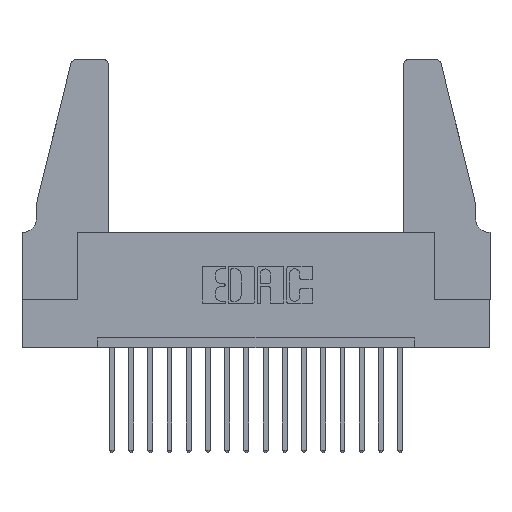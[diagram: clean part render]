
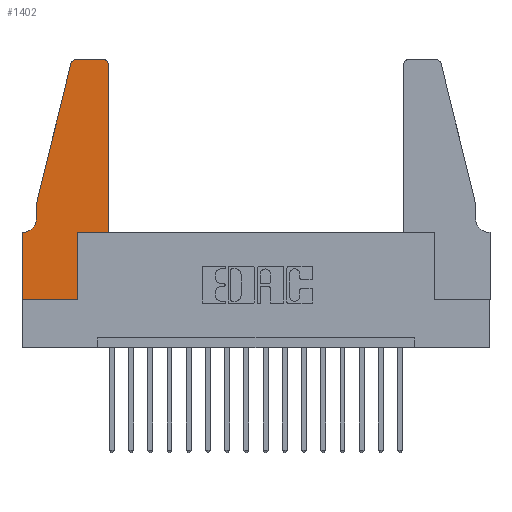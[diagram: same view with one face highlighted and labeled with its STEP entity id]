
A CAD part, top view. The second image highlights one B-rep face of the part: STEP entity #1402.
In plain terms, the highlighted planar face has unit normal (0, 0, 1).
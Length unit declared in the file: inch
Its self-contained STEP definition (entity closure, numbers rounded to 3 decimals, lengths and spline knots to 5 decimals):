
#218 = CARTESIAN_POINT ( 'NONE',  ( 0.25487, 1.22718, 0.37 ) ) ;
#246 = CIRCLE ( 'NONE', #5915, 0.03 ) ;
#632 = CARTESIAN_POINT ( 'NONE',  ( 0.4505, 0.35, 0.37 ) ) ;
#661 = LINE ( 'NONE', #895, #12252 ) ;
#686 = DIRECTION ( 'NONE',  ( -1., 0., 0. ) ) ;
#746 = DIRECTION ( 'NONE',  ( 1., 0., 0. ) ) ;
#895 = CARTESIAN_POINT ( 'NONE',  ( 0.0755, 0.35, 0.37 ) ) ;
#911 = VERTEX_POINT ( 'NONE', #13618 ) ;
#955 = CARTESIAN_POINT ( 'NONE',  ( 0.4205, 1.25, 0.37 ) ) ;
#1237 = CARTESIAN_POINT ( 'NONE',  ( 0.2865, 0.35, 0.37 ) ) ;
#1300 = DIRECTION ( 'NONE',  ( 0., 1., 0. ) ) ;
#1331 = EDGE_CURVE ( 'NONE', #10285, #3420, #5585, .T. ) ;
#1402 = ADVANCED_FACE ( 'NONE', ( #6008 ), #6118, .T. ) ;
#1501 = AXIS2_PLACEMENT_3D ( 'NONE', #3945, #5365, #5614 ) ;
#1996 = CARTESIAN_POINT ( 'NONE',  ( 0.0055, 0.42, 0.37 ) ) ;
#2020 = LINE ( 'NONE', #7307, #12555 ) ;
#3420 = VERTEX_POINT ( 'NONE', #8411 ) ;
#3944 = EDGE_CURVE ( 'NONE', #3420, #10377, #2020, .T. ) ;
#3945 = CARTESIAN_POINT ( 'NONE',  ( 0.284, 1.22, 0.37 ) ) ;
#4364 = DIRECTION ( 'NONE',  ( 0., -1., 0. ) ) ;
#4513 = VERTEX_POINT ( 'NONE', #7907 ) ;
#4606 = DIRECTION ( 'NONE',  ( 1., 0., 0. ) ) ;
#4682 = VERTEX_POINT ( 'NONE', #5174 ) ;
#4946 = EDGE_CURVE ( 'NONE', #10165, #10457, #15921, .T. ) ;
#5174 = CARTESIAN_POINT ( 'NONE',  ( 0.4505, 1.22, 0.37 ) ) ;
#5352 = VERTEX_POINT ( 'NONE', #11064 ) ;
#5365 = DIRECTION ( 'NONE',  ( 0., 0., 1. ) ) ;
#5369 = LINE ( 'NONE', #7234, #12212 ) ;
#5465 = ORIENTED_EDGE ( 'NONE', *, *, #4946, .T. ) ;
#5471 = VERTEX_POINT ( 'NONE', #955 ) ;
#5585 = LINE ( 'NONE', #10132, #12208 ) ;
#5614 = DIRECTION ( 'NONE',  ( 1., 0., 0. ) ) ;
#5915 = AXIS2_PLACEMENT_3D ( 'NONE', #13156, #6268, #15820 ) ;
#5952 = DIRECTION ( 'NONE',  ( -1., 0., 0. ) ) ;
#5994 = VERTEX_POINT ( 'NONE', #632 ) ;
#6008 = FACE_OUTER_BOUND ( 'NONE', #15232, .T. ) ;
#6050 = DIRECTION ( 'NONE',  ( 0., -1., 0. ) ) ;
#6091 = EDGE_CURVE ( 'NONE', #4513, #5352, #15668, .T. ) ;
#6118 = PLANE ( 'NONE',  #15606 ) ;
#6236 = DIRECTION ( 'NONE',  ( 0., 0., -1. ) ) ;
#6268 = DIRECTION ( 'NONE',  ( 0., 0., 1. ) ) ;
#6498 = LINE ( 'NONE', #13769, #12497 ) ;
#7151 = CARTESIAN_POINT ( 'NONE',  ( 0.0755, 0.5, 0.37 ) ) ;
#7234 = CARTESIAN_POINT ( 'NONE',  ( 0.2605, 1.25, 0.37 ) ) ;
#7270 = EDGE_CURVE ( 'NONE', #4682, #5471, #246, .T. ) ;
#7307 = CARTESIAN_POINT ( 'NONE',  ( 0., 0., 0.37 ) ) ;
#7512 = ORIENTED_EDGE ( 'NONE', *, *, #15019, .T. ) ;
#7577 = CARTESIAN_POINT ( 'NONE',  ( 0., 0.35, 0.37 ) ) ;
#7890 = ORIENTED_EDGE ( 'NONE', *, *, #8281, .T. ) ;
#7907 = CARTESIAN_POINT ( 'NONE',  ( 0.0755, 0.5, 0.37 ) ) ;
#8196 = ORIENTED_EDGE ( 'NONE', *, *, #8387, .T. ) ;
#8281 = EDGE_CURVE ( 'NONE', #5471, #10165, #5369, .T. ) ;
#8378 = VECTOR ( 'NONE', #6050, 39.37008 ) ;
#8387 = EDGE_CURVE ( 'NONE', #9005, #5994, #14546, .T. ) ;
#8411 = CARTESIAN_POINT ( 'NONE',  ( 0., 0., 0.37 ) ) ;
#8849 = CARTESIAN_POINT ( 'NONE',  ( 0.4505, 0.35, 0.37 ) ) ;
#8960 = DIRECTION ( 'NONE',  ( 0., 0., 1. ) ) ;
#9005 = VERTEX_POINT ( 'NONE', #15796 ) ;
#9134 = CARTESIAN_POINT ( 'NONE',  ( 0.284, 1.25, 0.37 ) ) ;
#9486 = CARTESIAN_POINT ( 'NONE',  ( 0.2865, 0., 0.37 ) ) ;
#9687 = DIRECTION ( 'NONE',  ( 0., 1., 0. ) ) ;
#10042 = ORIENTED_EDGE ( 'NONE', *, *, #16194, .T. ) ;
#10132 = CARTESIAN_POINT ( 'NONE',  ( 0., 0., 0.37 ) ) ;
#10165 = VERTEX_POINT ( 'NONE', #9134 ) ;
#10285 = VERTEX_POINT ( 'NONE', #12871 ) ;
#10377 = VERTEX_POINT ( 'NONE', #9486 ) ;
#10457 = VERTEX_POINT ( 'NONE', #218 ) ;
#10514 = LINE ( 'NONE', #17068, #16288 ) ;
#10724 = ORIENTED_EDGE ( 'NONE', *, *, #15598, .T. ) ;
#10928 = VECTOR ( 'NONE', #4606, 39.37008 ) ;
#11064 = CARTESIAN_POINT ( 'NONE',  ( 0.0755, 0.42, 0.37 ) ) ;
#11336 = VECTOR ( 'NONE', #1300, 39.37008 ) ;
#11367 = ORIENTED_EDGE ( 'NONE', *, *, #7270, .T. ) ;
#11774 = LINE ( 'NONE', #1237, #11336 ) ;
#12208 = VECTOR ( 'NONE', #4364, 39.37008 ) ;
#12212 = VECTOR ( 'NONE', #5952, 39.37008 ) ;
#12252 = VECTOR ( 'NONE', #13246, 39.37008 ) ;
#12497 = VECTOR ( 'NONE', #9687, 39.37008 ) ;
#12555 = VECTOR ( 'NONE', #14224, 39.37008 ) ;
#12871 = CARTESIAN_POINT ( 'NONE',  ( 0., 0.35, 0.37 ) ) ;
#13049 = ORIENTED_EDGE ( 'NONE', *, *, #6091, .T. ) ;
#13156 = CARTESIAN_POINT ( 'NONE',  ( 0.4205, 1.22, 0.37 ) ) ;
#13246 = DIRECTION ( 'NONE',  ( -1., 0., 0. ) ) ;
#13420 = AXIS2_PLACEMENT_3D ( 'NONE', #1996, #6236, #686 ) ;
#13618 = CARTESIAN_POINT ( 'NONE',  ( 0.0055, 0.35, 0.37 ) ) ;
#13760 = CIRCLE ( 'NONE', #13420, 0.07 ) ;
#13769 = CARTESIAN_POINT ( 'NONE',  ( 0.4505, 0.35, 0.37 ) ) ;
#14224 = DIRECTION ( 'NONE',  ( 1., 0., 0. ) ) ;
#14310 = EDGE_CURVE ( 'NONE', #5994, #4682, #6498, .T. ) ;
#14546 = LINE ( 'NONE', #8849, #10928 ) ;
#14548 = ORIENTED_EDGE ( 'NONE', *, *, #14310, .T. ) ;
#14785 = ORIENTED_EDGE ( 'NONE', *, *, #3944, .T. ) ;
#15019 = EDGE_CURVE ( 'NONE', #911, #10285, #661, .T. ) ;
#15232 = EDGE_LOOP ( 'NONE', ( #7890, #5465, #10724, #13049, #15816, #7512, #17011, #14785, #10042, #8196, #14548, #11367 ) ) ;
#15402 = EDGE_CURVE ( 'NONE', #5352, #911, #13760, .T. ) ;
#15598 = EDGE_CURVE ( 'NONE', #10457, #4513, #10514, .T. ) ;
#15606 = AXIS2_PLACEMENT_3D ( 'NONE', #7577, #8960, #746 ) ;
#15648 = DIRECTION ( 'NONE',  ( -0.239, -0.971, 0. ) ) ;
#15668 = LINE ( 'NONE', #7151, #8378 ) ;
#15796 = CARTESIAN_POINT ( 'NONE',  ( 0.2865, 0.35, 0.37 ) ) ;
#15816 = ORIENTED_EDGE ( 'NONE', *, *, #15402, .T. ) ;
#15820 = DIRECTION ( 'NONE',  ( 1., 0., 0. ) ) ;
#15921 = CIRCLE ( 'NONE', #1501, 0.03 ) ;
#16194 = EDGE_CURVE ( 'NONE', #10377, #9005, #11774, .T. ) ;
#16288 = VECTOR ( 'NONE', #15648, 39.37008 ) ;
#17011 = ORIENTED_EDGE ( 'NONE', *, *, #1331, .T. ) ;
#17068 = CARTESIAN_POINT ( 'NONE',  ( 0.0755, 0.5, 0.37 ) ) ;
